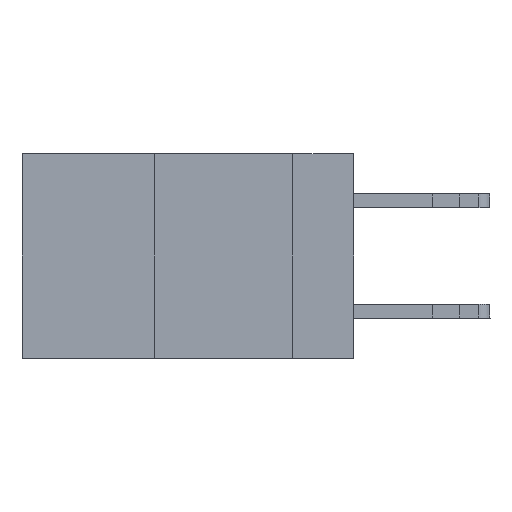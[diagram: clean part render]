
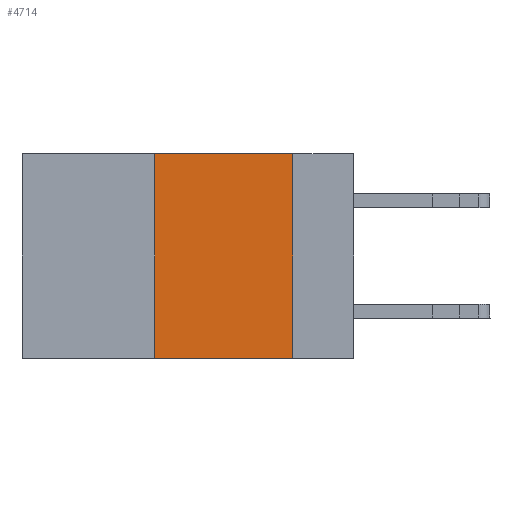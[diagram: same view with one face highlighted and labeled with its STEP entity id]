
A CAD part, left-side view. The second image highlights one B-rep face of the part: STEP entity #4714.
In plain terms, the highlighted planar face has unit normal (-1, 0, 0).
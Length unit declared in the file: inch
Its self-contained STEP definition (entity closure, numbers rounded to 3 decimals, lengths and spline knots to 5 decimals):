
#656 = DIRECTION ( 'NONE',  ( 0., -1., 0. ) ) ;
#1008 = LINE ( 'NONE', #17328, #15160 ) ;
#2143 = DIRECTION ( 'NONE',  ( 0., 0., 1. ) ) ;
#2155 = PLANE ( 'NONE',  #15545 ) ;
#3301 = ORIENTED_EDGE ( 'NONE', *, *, #12621, .F. ) ;
#3664 = ORIENTED_EDGE ( 'NONE', *, *, #3712, .F. ) ;
#3712 = EDGE_CURVE ( 'NONE', #16452, #16080, #15104, .T. ) ;
#3752 = VECTOR ( 'NONE', #4044, 39.37008 ) ;
#4044 = DIRECTION ( 'NONE',  ( 0., -1., 0. ) ) ;
#4714 = ADVANCED_FACE ( 'NONE', ( #14308 ), #2155, .F. ) ;
#5619 = EDGE_LOOP ( 'NONE', ( #3664, #7703, #3301, #10806 ) ) ;
#6496 = EDGE_CURVE ( 'NONE', #10502, #16452, #7708, .T. ) ;
#6708 = CARTESIAN_POINT ( 'NONE',  ( 0., 0.6, 0. ) ) ;
#7377 = CARTESIAN_POINT ( 'NONE',  ( 0., 0.11, 0. ) ) ;
#7578 = VECTOR ( 'NONE', #9029, 39.37008 ) ;
#7703 = ORIENTED_EDGE ( 'NONE', *, *, #6496, .F. ) ;
#7708 = LINE ( 'NONE', #14815, #3752 ) ;
#8263 = CARTESIAN_POINT ( 'NONE',  ( 0., 0.36, 0. ) ) ;
#9029 = DIRECTION ( 'NONE',  ( 0., 0., -1. ) ) ;
#9588 = DIRECTION ( 'NONE',  ( 0., 0., -1. ) ) ;
#10502 = VERTEX_POINT ( 'NONE', #8263 ) ;
#10621 = CARTESIAN_POINT ( 'NONE',  ( 0., 0.11, 0. ) ) ;
#10806 = ORIENTED_EDGE ( 'NONE', *, *, #13490, .T. ) ;
#12429 = VECTOR ( 'NONE', #656, 39.37008 ) ;
#12444 = VERTEX_POINT ( 'NONE', #17044 ) ;
#12621 = EDGE_CURVE ( 'NONE', #12444, #10502, #1008, .T. ) ;
#13460 = CARTESIAN_POINT ( 'NONE',  ( 0., 0.11, -0.37 ) ) ;
#13490 = EDGE_CURVE ( 'NONE', #12444, #16080, #15838, .T. ) ;
#14308 = FACE_OUTER_BOUND ( 'NONE', #5619, .T. ) ;
#14815 = CARTESIAN_POINT ( 'NONE',  ( 0., 0.6, 0. ) ) ;
#15104 = LINE ( 'NONE', #10621, #7578 ) ;
#15160 = VECTOR ( 'NONE', #2143, 39.37008 ) ;
#15545 = AXIS2_PLACEMENT_3D ( 'NONE', #6708, #17391, #9588 ) ;
#15838 = LINE ( 'NONE', #17422, #12429 ) ;
#16080 = VERTEX_POINT ( 'NONE', #13460 ) ;
#16452 = VERTEX_POINT ( 'NONE', #7377 ) ;
#17044 = CARTESIAN_POINT ( 'NONE',  ( 0., 0.36, -0.37 ) ) ;
#17328 = CARTESIAN_POINT ( 'NONE',  ( 0., 0.36, 0. ) ) ;
#17391 = DIRECTION ( 'NONE',  ( 1., 0., 0. ) ) ;
#17422 = CARTESIAN_POINT ( 'NONE',  ( 0., 0.6, -0.37 ) ) ;
